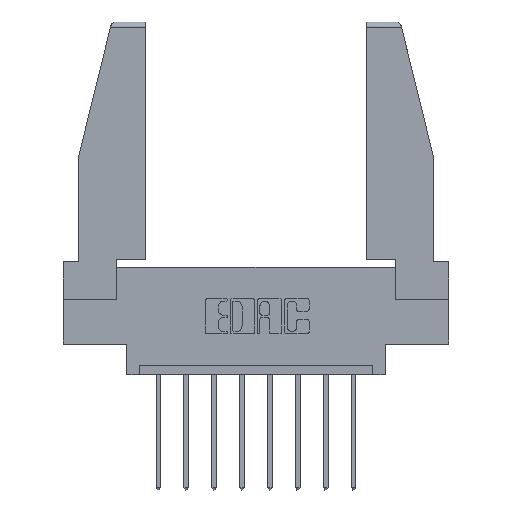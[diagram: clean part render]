
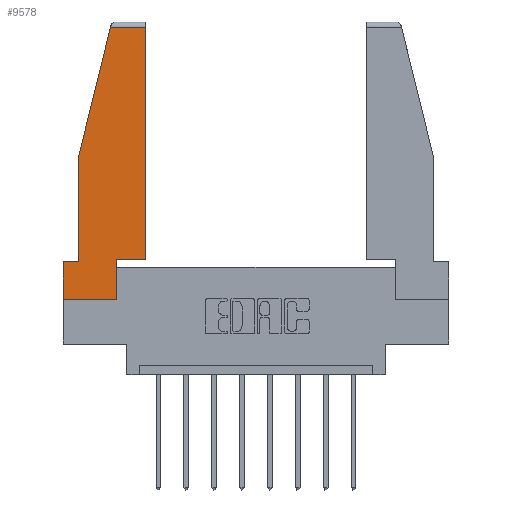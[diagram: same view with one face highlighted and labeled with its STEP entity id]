
A CAD part, top view. The second image highlights one B-rep face of the part: STEP entity #9578.
In plain terms, the highlighted planar face has unit normal (0, 0, 1).
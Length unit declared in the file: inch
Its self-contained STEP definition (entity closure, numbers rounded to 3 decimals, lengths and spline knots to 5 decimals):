
#52 = ORIENTED_EDGE ( 'NONE', *, *, #9178, .T. ) ;
#57 = PLANE ( 'NONE',  #8095 ) ;
#62 = VECTOR ( 'NONE', #9497, 39.37008 ) ;
#179 = VECTOR ( 'NONE', #11091, 39.37008 ) ;
#436 = CARTESIAN_POINT ( 'NONE',  ( 0.086, 0.8, 0. ) ) ;
#723 = DIRECTION ( 'NONE',  ( 0., 1., 0. ) ) ;
#840 = DIRECTION ( 'NONE',  ( 0., -1., 0. ) ) ;
#944 = VERTEX_POINT ( 'NONE', #6730 ) ;
#1237 = ORIENTED_EDGE ( 'NONE', *, *, #12632, .T. ) ;
#1552 = DIRECTION ( 'NONE',  ( -1., 0., 0. ) ) ;
#1619 = CARTESIAN_POINT ( 'NONE',  ( 0.297, 0., 0. ) ) ;
#1677 = LINE ( 'NONE', #1619, #3560 ) ;
#1702 = VERTEX_POINT ( 'NONE', #12864 ) ;
#1848 = DIRECTION ( 'NONE',  ( 1., 0., 0. ) ) ;
#1950 = EDGE_CURVE ( 'NONE', #11479, #11018, #11390, .T. ) ;
#2071 = CARTESIAN_POINT ( 'NONE',  ( 0., 0.21, 0. ) ) ;
#2172 = EDGE_LOOP ( 'NONE', ( #8054, #12280, #7835, #12265, #6323, #8769, #52, #1237, #7049 ) ) ;
#2231 = FACE_OUTER_BOUND ( 'NONE', #2172, .T. ) ;
#2405 = LINE ( 'NONE', #7893, #9004 ) ;
#2742 = CARTESIAN_POINT ( 'NONE',  ( 0.2636, 1.52, 0. ) ) ;
#2803 = CARTESIAN_POINT ( 'NONE',  ( 0.271, 1.55, 0. ) ) ;
#3022 = EDGE_CURVE ( 'NONE', #11018, #5536, #2405, .T. ) ;
#3238 = VECTOR ( 'NONE', #1552, 39.37008 ) ;
#3516 = CARTESIAN_POINT ( 'NONE',  ( 0.461, 0.223, 0. ) ) ;
#3528 = CARTESIAN_POINT ( 'NONE',  ( 0., 1.52, 0. ) ) ;
#3560 = VECTOR ( 'NONE', #723, 39.37008 ) ;
#4080 = CARTESIAN_POINT ( 'NONE',  ( 0., 0., 0. ) ) ;
#4233 = EDGE_CURVE ( 'NONE', #10876, #4574, #4241, .T. ) ;
#4241 = LINE ( 'NONE', #7957, #179 ) ;
#4286 = VECTOR ( 'NONE', #12909, 39.37008 ) ;
#4384 = VERTEX_POINT ( 'NONE', #11225 ) ;
#4574 = VERTEX_POINT ( 'NONE', #5144 ) ;
#4867 = DIRECTION ( 'NONE',  ( 0., -1., 0. ) ) ;
#4893 = LINE ( 'NONE', #5894, #11804 ) ;
#5066 = LINE ( 'NONE', #8889, #5226 ) ;
#5144 = CARTESIAN_POINT ( 'NONE',  ( 0.461, 1.52, 0. ) ) ;
#5226 = VECTOR ( 'NONE', #1848, 39.37008 ) ;
#5536 = VERTEX_POINT ( 'NONE', #11170 ) ;
#5894 = CARTESIAN_POINT ( 'NONE',  ( 0., 0.21, 0. ) ) ;
#6001 = DIRECTION ( 'NONE',  ( 0., 0., 1. ) ) ;
#6047 = CARTESIAN_POINT ( 'NONE',  ( 0., 0., 0. ) ) ;
#6240 = LINE ( 'NONE', #3528, #3238 ) ;
#6323 = ORIENTED_EDGE ( 'NONE', *, *, #8632, .T. ) ;
#6730 = CARTESIAN_POINT ( 'NONE',  ( 0., 0., 0. ) ) ;
#7049 = ORIENTED_EDGE ( 'NONE', *, *, #9491, .T. ) ;
#7339 = DIRECTION ( 'NONE',  ( 1., 0., 0. ) ) ;
#7835 = ORIENTED_EDGE ( 'NONE', *, *, #1950, .T. ) ;
#7893 = CARTESIAN_POINT ( 'NONE',  ( 0.086, 0.8, 0. ) ) ;
#7957 = CARTESIAN_POINT ( 'NONE',  ( 0.461, 0.223, 0. ) ) ;
#8054 = ORIENTED_EDGE ( 'NONE', *, *, #4233, .T. ) ;
#8095 = AXIS2_PLACEMENT_3D ( 'NONE', #4080, #6001, #7339 ) ;
#8225 = LINE ( 'NONE', #8799, #62 ) ;
#8632 = EDGE_CURVE ( 'NONE', #5536, #9568, #8225, .T. ) ;
#8739 = DIRECTION ( 'NONE',  ( -0.239, -0.971, 0. ) ) ;
#8769 = ORIENTED_EDGE ( 'NONE', *, *, #9740, .T. ) ;
#8799 = CARTESIAN_POINT ( 'NONE',  ( 0., 0.21, 0. ) ) ;
#8889 = CARTESIAN_POINT ( 'NONE',  ( 0.297, 0.223, 0. ) ) ;
#9004 = VECTOR ( 'NONE', #840, 39.37008 ) ;
#9178 = EDGE_CURVE ( 'NONE', #944, #1702, #12570, .T. ) ;
#9491 = EDGE_CURVE ( 'NONE', #4384, #10876, #5066, .T. ) ;
#9497 = DIRECTION ( 'NONE',  ( -1., 0., 0. ) ) ;
#9568 = VERTEX_POINT ( 'NONE', #2071 ) ;
#9578 = ADVANCED_FACE ( 'NONE', ( #2231 ), #57, .T. ) ;
#9740 = EDGE_CURVE ( 'NONE', #9568, #944, #4893, .T. ) ;
#10773 = VECTOR ( 'NONE', #8739, 39.37008 ) ;
#10876 = VERTEX_POINT ( 'NONE', #3516 ) ;
#11018 = VERTEX_POINT ( 'NONE', #436 ) ;
#11091 = DIRECTION ( 'NONE',  ( 0., 1., 0. ) ) ;
#11170 = CARTESIAN_POINT ( 'NONE',  ( 0.086, 0.21, 0. ) ) ;
#11225 = CARTESIAN_POINT ( 'NONE',  ( 0.297, 0.223, 0. ) ) ;
#11390 = LINE ( 'NONE', #2803, #10773 ) ;
#11479 = VERTEX_POINT ( 'NONE', #2742 ) ;
#11804 = VECTOR ( 'NONE', #4867, 39.37008 ) ;
#12265 = ORIENTED_EDGE ( 'NONE', *, *, #3022, .T. ) ;
#12280 = ORIENTED_EDGE ( 'NONE', *, *, #12951, .T. ) ;
#12570 = LINE ( 'NONE', #6047, #4286 ) ;
#12632 = EDGE_CURVE ( 'NONE', #1702, #4384, #1677, .T. ) ;
#12864 = CARTESIAN_POINT ( 'NONE',  ( 0.297, 0., 0. ) ) ;
#12909 = DIRECTION ( 'NONE',  ( 1., 0., 0. ) ) ;
#12951 = EDGE_CURVE ( 'NONE', #4574, #11479, #6240, .T. ) ;
